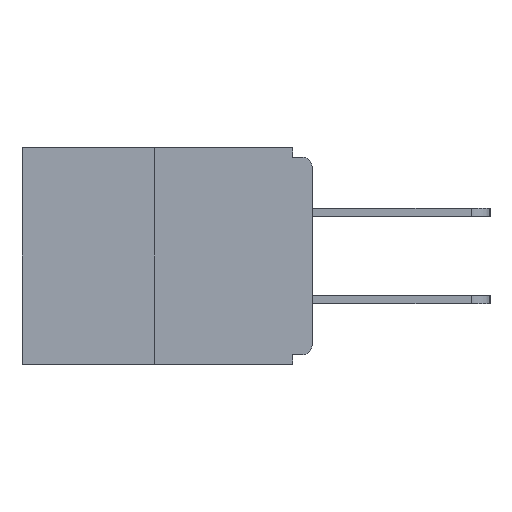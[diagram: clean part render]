
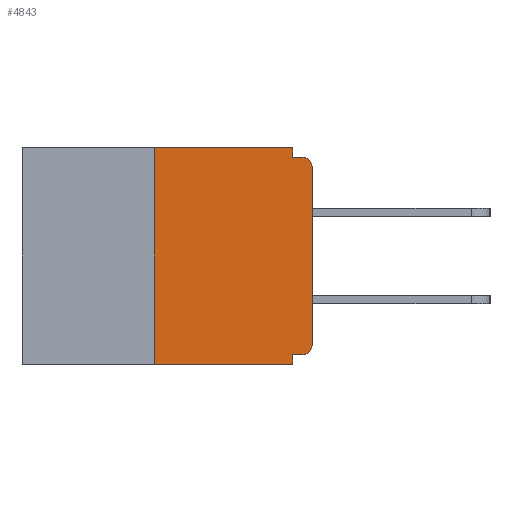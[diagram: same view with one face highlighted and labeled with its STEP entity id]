
A CAD part, left-side view. The second image highlights one B-rep face of the part: STEP entity #4843.
In plain terms, the highlighted planar face has unit normal (-1, 0, 0).
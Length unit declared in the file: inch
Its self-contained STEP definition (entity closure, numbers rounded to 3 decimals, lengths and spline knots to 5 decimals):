
#232 = DIRECTION ( 'NONE',  ( 0., 0., -1. ) ) ;
#461 = ORIENTED_EDGE ( 'NONE', *, *, #15120, .F. ) ;
#610 = ORIENTED_EDGE ( 'NONE', *, *, #8926, .T. ) ;
#931 = DIRECTION ( 'NONE',  ( 0., 0., -1. ) ) ;
#1073 = VERTEX_POINT ( 'NONE', #12024 ) ;
#1152 = LINE ( 'NONE', #14689, #13594 ) ;
#1673 = DIRECTION ( 'NONE',  ( -1., 0., 0. ) ) ;
#1709 = DIRECTION ( 'NONE',  ( -1., 0., 0. ) ) ;
#2092 = CARTESIAN_POINT ( 'NONE',  ( 0., 0.25, -0.343 ) ) ;
#2120 = FACE_OUTER_BOUND ( 'NONE', #10748, .T. ) ;
#2265 = DIRECTION ( 'NONE',  ( 0., -1., 0. ) ) ;
#2592 = VERTEX_POINT ( 'NONE', #14996 ) ;
#3148 = CARTESIAN_POINT ( 'NONE',  ( 0., 0.031, -0.015 ) ) ;
#4177 = VECTOR ( 'NONE', #8880, 39.37008 ) ;
#4371 = DIRECTION ( 'NONE',  ( 0., -1., 0. ) ) ;
#4620 = DIRECTION ( 'NONE',  ( 0., 0., -1. ) ) ;
#4843 = ADVANCED_FACE ( 'NONE', ( #2120 ), #25513, .F. ) ;
#5300 = VERTEX_POINT ( 'NONE', #7957 ) ;
#6432 = ORIENTED_EDGE ( 'NONE', *, *, #24160, .F. ) ;
#6631 = AXIS2_PLACEMENT_3D ( 'NONE', #13796, #1673, #9999 ) ;
#6904 = CARTESIAN_POINT ( 'NONE',  ( 0., 0., 0. ) ) ;
#6982 = VECTOR ( 'NONE', #4620, 39.37008 ) ;
#7082 = VERTEX_POINT ( 'NONE', #3148 ) ;
#7607 = DIRECTION ( 'NONE',  ( 0., 0., -1. ) ) ;
#7779 = EDGE_CURVE ( 'NONE', #13845, #5300, #8396, .T. ) ;
#7957 = CARTESIAN_POINT ( 'NONE',  ( 0., 0.031, -0.328 ) ) ;
#8211 = VECTOR ( 'NONE', #20831, 39.37008 ) ;
#8355 = CARTESIAN_POINT ( 'NONE',  ( 0., 0., -0.015 ) ) ;
#8396 = LINE ( 'NONE', #15759, #18607 ) ;
#8770 = VECTOR ( 'NONE', #2265, 39.37008 ) ;
#8812 = ORIENTED_EDGE ( 'NONE', *, *, #7779, .F. ) ;
#8880 = DIRECTION ( 'NONE',  ( 0., 0., 1. ) ) ;
#8926 = EDGE_CURVE ( 'NONE', #21625, #14905, #1152, .T. ) ;
#8954 = EDGE_CURVE ( 'NONE', #5300, #14905, #21588, .T. ) ;
#9680 = ORIENTED_EDGE ( 'NONE', *, *, #15294, .T. ) ;
#9848 = CARTESIAN_POINT ( 'NONE',  ( 0., 0.015, -0.03 ) ) ;
#9999 = DIRECTION ( 'NONE',  ( 0., 0., -1. ) ) ;
#10441 = CARTESIAN_POINT ( 'NONE',  ( 0., 0.031, 0. ) ) ;
#10748 = EDGE_LOOP ( 'NONE', ( #15058, #461, #610, #19199, #8812, #14772, #13258, #9680, #18730, #6432 ) ) ;
#11133 = CARTESIAN_POINT ( 'NONE',  ( 0., 0.46, 0. ) ) ;
#11329 = EDGE_CURVE ( 'NONE', #13845, #1073, #24657, .T. ) ;
#12024 = CARTESIAN_POINT ( 'NONE',  ( 0., 0., -0.313 ) ) ;
#12166 = CIRCLE ( 'NONE', #12340, 0.015 ) ;
#12299 = DIRECTION ( 'NONE',  ( 0., 1., 0. ) ) ;
#12340 = AXIS2_PLACEMENT_3D ( 'NONE', #9848, #1709, #7607 ) ;
#13216 = VERTEX_POINT ( 'NONE', #13485 ) ;
#13258 = ORIENTED_EDGE ( 'NONE', *, *, #17635, .T. ) ;
#13485 = CARTESIAN_POINT ( 'NONE',  ( 0., 0.25, 0. ) ) ;
#13594 = VECTOR ( 'NONE', #4371, 39.37008 ) ;
#13796 = CARTESIAN_POINT ( 'NONE',  ( 0., 0.015, -0.313 ) ) ;
#13845 = VERTEX_POINT ( 'NONE', #26301 ) ;
#14621 = LINE ( 'NONE', #10441, #6982 ) ;
#14689 = CARTESIAN_POINT ( 'NONE',  ( 0., 0.46, -0.343 ) ) ;
#14772 = ORIENTED_EDGE ( 'NONE', *, *, #11329, .T. ) ;
#14905 = VERTEX_POINT ( 'NONE', #24326 ) ;
#14996 = CARTESIAN_POINT ( 'NONE',  ( 0., 0., -0.03 ) ) ;
#15042 = DIRECTION ( 'NONE',  ( 0., -1., 0. ) ) ;
#15058 = ORIENTED_EDGE ( 'NONE', *, *, #21989, .F. ) ;
#15120 = EDGE_CURVE ( 'NONE', #21625, #13216, #24481, .T. ) ;
#15294 = EDGE_CURVE ( 'NONE', #2592, #15896, #12166, .T. ) ;
#15759 = CARTESIAN_POINT ( 'NONE',  ( 0., 0., -0.328 ) ) ;
#15896 = VERTEX_POINT ( 'NONE', #17735 ) ;
#15980 = EDGE_CURVE ( 'NONE', #7082, #15896, #26014, .T. ) ;
#16030 = VECTOR ( 'NONE', #15042, 39.37008 ) ;
#17635 = EDGE_CURVE ( 'NONE', #1073, #2592, #24291, .T. ) ;
#17735 = CARTESIAN_POINT ( 'NONE',  ( 0., 0.015, -0.015 ) ) ;
#18607 = VECTOR ( 'NONE', #12299, 39.37008 ) ;
#18730 = ORIENTED_EDGE ( 'NONE', *, *, #15980, .F. ) ;
#18931 = VERTEX_POINT ( 'NONE', #25637 ) ;
#19199 = ORIENTED_EDGE ( 'NONE', *, *, #8954, .F. ) ;
#20602 = CARTESIAN_POINT ( 'NONE',  ( 0., 0.031, -0.343 ) ) ;
#20831 = DIRECTION ( 'NONE',  ( 0., 0., 1. ) ) ;
#21151 = LINE ( 'NONE', #23163, #16030 ) ;
#21588 = LINE ( 'NONE', #20602, #23175 ) ;
#21625 = VERTEX_POINT ( 'NONE', #2092 ) ;
#21989 = EDGE_CURVE ( 'NONE', #13216, #18931, #21151, .T. ) ;
#23163 = CARTESIAN_POINT ( 'NONE',  ( 0., 0.46, 0. ) ) ;
#23175 = VECTOR ( 'NONE', #232, 39.37008 ) ;
#24160 = EDGE_CURVE ( 'NONE', #18931, #7082, #14621, .T. ) ;
#24291 = LINE ( 'NONE', #6904, #4177 ) ;
#24326 = CARTESIAN_POINT ( 'NONE',  ( 0., 0.031, -0.343 ) ) ;
#24481 = LINE ( 'NONE', #24862, #8211 ) ;
#24657 = CIRCLE ( 'NONE', #6631, 0.015 ) ;
#24862 = CARTESIAN_POINT ( 'NONE',  ( 0., 0.25, 0. ) ) ;
#25246 = DIRECTION ( 'NONE',  ( 1., 0., 0. ) ) ;
#25259 = AXIS2_PLACEMENT_3D ( 'NONE', #11133, #25246, #931 ) ;
#25513 = PLANE ( 'NONE',  #25259 ) ;
#25637 = CARTESIAN_POINT ( 'NONE',  ( 0., 0.031, 0. ) ) ;
#26014 = LINE ( 'NONE', #8355, #8770 ) ;
#26301 = CARTESIAN_POINT ( 'NONE',  ( 0., 0.015, -0.328 ) ) ;
